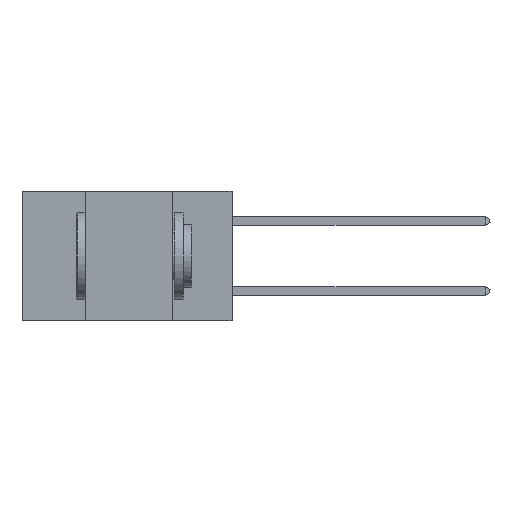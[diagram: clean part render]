
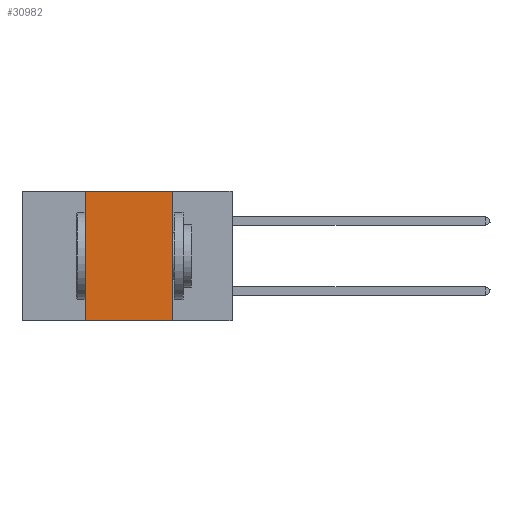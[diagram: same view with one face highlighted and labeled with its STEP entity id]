
A CAD part, left-side view. The second image highlights one B-rep face of the part: STEP entity #30982.
In plain terms, the highlighted planar face has unit normal (-1, 0, 0).
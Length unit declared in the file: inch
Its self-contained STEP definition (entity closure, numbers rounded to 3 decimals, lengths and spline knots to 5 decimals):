
#1415 = LINE ( 'NONE', #16790, #26282 ) ;
#2317 = CARTESIAN_POINT ( 'NONE',  ( 0., 0.6, 0. ) ) ;
#2474 = VERTEX_POINT ( 'NONE', #12008 ) ;
#2972 = CARTESIAN_POINT ( 'NONE',  ( 0., 0.6, -0.37 ) ) ;
#3171 = LINE ( 'NONE', #2317, #30967 ) ;
#6942 = CARTESIAN_POINT ( 'NONE',  ( 0., 0.6, 0. ) ) ;
#7665 = VERTEX_POINT ( 'NONE', #22841 ) ;
#8163 = CARTESIAN_POINT ( 'NONE',  ( 0., 0.42, 0. ) ) ;
#8236 = FACE_OUTER_BOUND ( 'NONE', #27855, .T. ) ;
#10363 = DIRECTION ( 'NONE',  ( 0., -1., 0. ) ) ;
#10557 = DIRECTION ( 'NONE',  ( 0., 0., 1. ) ) ;
#11243 = DIRECTION ( 'NONE',  ( 0., 0., -1. ) ) ;
#12008 = CARTESIAN_POINT ( 'NONE',  ( 0., 0.42, 0. ) ) ;
#12623 = CARTESIAN_POINT ( 'NONE',  ( 0., 0.42, -0.37 ) ) ;
#13457 = LINE ( 'NONE', #2972, #18522 ) ;
#14287 = ORIENTED_EDGE ( 'NONE', *, *, #23158, .F. ) ;
#14966 = DIRECTION ( 'NONE',  ( 1., 0., 0. ) ) ;
#15544 = EDGE_CURVE ( 'NONE', #20087, #7665, #13457, .T. ) ;
#16790 = CARTESIAN_POINT ( 'NONE',  ( 0., 0.17, 0. ) ) ;
#17578 = PLANE ( 'NONE',  #21419 ) ;
#18522 = VECTOR ( 'NONE', #19146, 39.37008 ) ;
#18606 = VECTOR ( 'NONE', #10557, 39.37008 ) ;
#19146 = DIRECTION ( 'NONE',  ( 0., -1., 0. ) ) ;
#19394 = ORIENTED_EDGE ( 'NONE', *, *, #15544, .T. ) ;
#20087 = VERTEX_POINT ( 'NONE', #12623 ) ;
#21419 = AXIS2_PLACEMENT_3D ( 'NONE', #6942, #14966, #28474 ) ;
#22841 = CARTESIAN_POINT ( 'NONE',  ( 0., 0.17, -0.37 ) ) ;
#23158 = EDGE_CURVE ( 'NONE', #20087, #2474, #30783, .T. ) ;
#25954 = EDGE_CURVE ( 'NONE', #30479, #7665, #1415, .T. ) ;
#26282 = VECTOR ( 'NONE', #11243, 39.37008 ) ;
#27855 = EDGE_LOOP ( 'NONE', ( #32363, #34079, #14287, #19394 ) ) ;
#28474 = DIRECTION ( 'NONE',  ( 0., 0., -1. ) ) ;
#30479 = VERTEX_POINT ( 'NONE', #33895 ) ;
#30783 = LINE ( 'NONE', #8163, #18606 ) ;
#30967 = VECTOR ( 'NONE', #10363, 39.37008 ) ;
#30982 = ADVANCED_FACE ( 'NONE', ( #8236 ), #17578, .F. ) ;
#31155 = EDGE_CURVE ( 'NONE', #2474, #30479, #3171, .T. ) ;
#32363 = ORIENTED_EDGE ( 'NONE', *, *, #25954, .F. ) ;
#33895 = CARTESIAN_POINT ( 'NONE',  ( 0., 0.17, 0. ) ) ;
#34079 = ORIENTED_EDGE ( 'NONE', *, *, #31155, .F. ) ;
